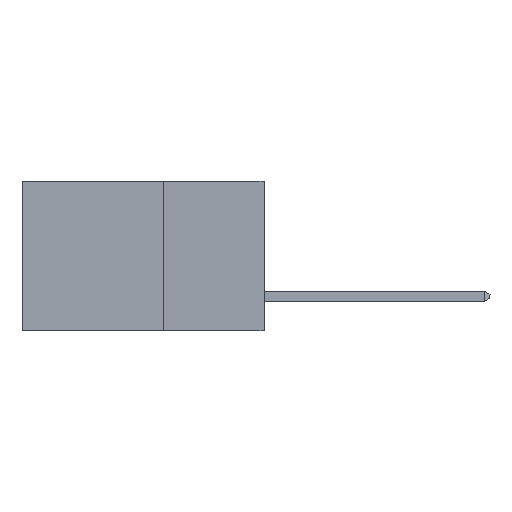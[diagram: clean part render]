
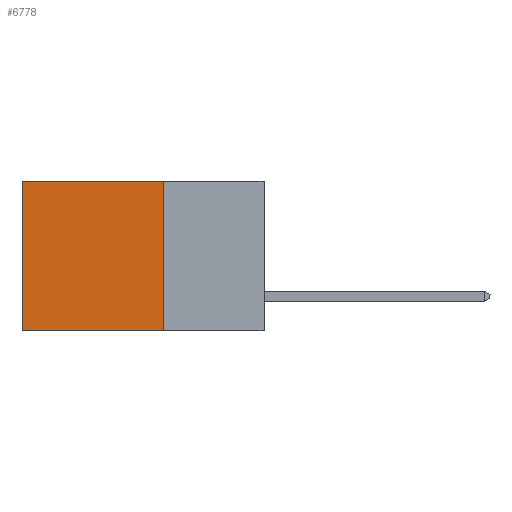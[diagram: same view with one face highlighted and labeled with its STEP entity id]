
A CAD part, left-side view. The second image highlights one B-rep face of the part: STEP entity #6778.
In plain terms, the highlighted planar face has unit normal (-1, 0, 0).
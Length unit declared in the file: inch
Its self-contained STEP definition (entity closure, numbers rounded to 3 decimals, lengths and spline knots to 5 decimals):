
#218 = CARTESIAN_POINT ( 'NONE',  ( 0.2615, 0.25, -0.37 ) ) ;
#259 = VECTOR ( 'NONE', #4806, 39.37008 ) ;
#793 = CARTESIAN_POINT ( 'NONE',  ( 0.2615, 0.6, -0.37 ) ) ;
#815 = ORIENTED_EDGE ( 'NONE', *, *, #5730, .T. ) ;
#829 = ORIENTED_EDGE ( 'NONE', *, *, #1254, .F. ) ;
#892 = LINE ( 'NONE', #3600, #6836 ) ;
#1254 = EDGE_CURVE ( 'NONE', #2614, #1857, #1387, .T. ) ;
#1387 = LINE ( 'NONE', #6136, #2691 ) ;
#1643 = EDGE_CURVE ( 'NONE', #8189, #2614, #3335, .T. ) ;
#1857 = VERTEX_POINT ( 'NONE', #793 ) ;
#2525 = EDGE_LOOP ( 'NONE', ( #815, #829, #2778, #8113 ) ) ;
#2614 = VERTEX_POINT ( 'NONE', #218 ) ;
#2691 = VECTOR ( 'NONE', #3304, 39.37008 ) ;
#2756 = PLANE ( 'NONE',  #4502 ) ;
#2778 = ORIENTED_EDGE ( 'NONE', *, *, #1643, .F. ) ;
#2784 = CARTESIAN_POINT ( 'NONE',  ( 0.2615, 0.25, 0. ) ) ;
#3304 = DIRECTION ( 'NONE',  ( 0., 1., 0. ) ) ;
#3335 = LINE ( 'NONE', #6037, #6006 ) ;
#3449 = EDGE_CURVE ( 'NONE', #8189, #8005, #5654, .T. ) ;
#3562 = DIRECTION ( 'NONE',  ( 1., 0., 0. ) ) ;
#3600 = CARTESIAN_POINT ( 'NONE',  ( 0.2615, 0.6, -0.37 ) ) ;
#4045 = DIRECTION ( 'NONE',  ( 0., 0., -1. ) ) ;
#4502 = AXIS2_PLACEMENT_3D ( 'NONE', #7478, #3562, #4045 ) ;
#4806 = DIRECTION ( 'NONE',  ( 0., 1., 0. ) ) ;
#5654 = LINE ( 'NONE', #2784, #259 ) ;
#5730 = EDGE_CURVE ( 'NONE', #8005, #1857, #892, .T. ) ;
#6006 = VECTOR ( 'NONE', #7343, 39.37008 ) ;
#6037 = CARTESIAN_POINT ( 'NONE',  ( 0.2615, 0.25, -0.37 ) ) ;
#6136 = CARTESIAN_POINT ( 'NONE',  ( 0.2615, 0.25, -0.37 ) ) ;
#6341 = DIRECTION ( 'NONE',  ( 0., 0., -1. ) ) ;
#6778 = ADVANCED_FACE ( 'NONE', ( #6801 ), #2756, .F. ) ;
#6801 = FACE_OUTER_BOUND ( 'NONE', #2525, .T. ) ;
#6836 = VECTOR ( 'NONE', #6341, 39.37008 ) ;
#7343 = DIRECTION ( 'NONE',  ( 0., 0., -1. ) ) ;
#7478 = CARTESIAN_POINT ( 'NONE',  ( 0.2615, 0.25, -0.37 ) ) ;
#8005 = VERTEX_POINT ( 'NONE', #8116 ) ;
#8113 = ORIENTED_EDGE ( 'NONE', *, *, #3449, .T. ) ;
#8116 = CARTESIAN_POINT ( 'NONE',  ( 0.2615, 0.6, 0. ) ) ;
#8177 = CARTESIAN_POINT ( 'NONE',  ( 0.2615, 0.25, 0. ) ) ;
#8189 = VERTEX_POINT ( 'NONE', #8177 ) ;
